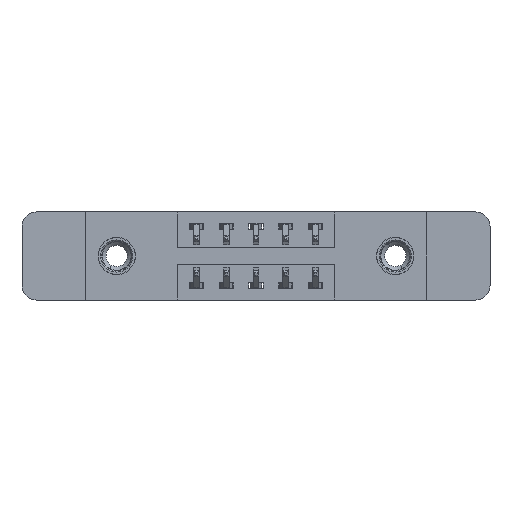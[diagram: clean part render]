
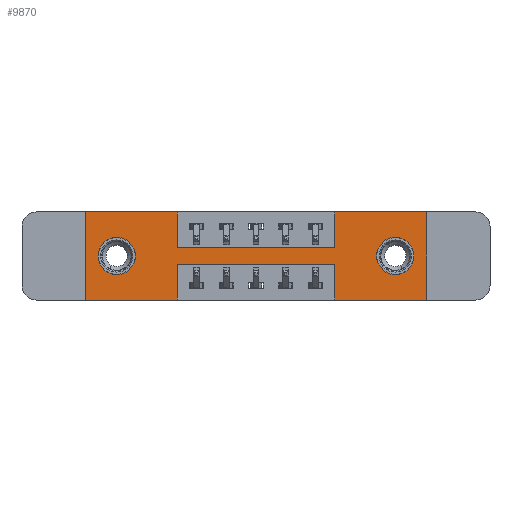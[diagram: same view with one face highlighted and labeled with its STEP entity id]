
A CAD part, front view. The second image highlights one B-rep face of the part: STEP entity #9870.
In plain terms, the highlighted planar face has unit normal (0, -1, 0).
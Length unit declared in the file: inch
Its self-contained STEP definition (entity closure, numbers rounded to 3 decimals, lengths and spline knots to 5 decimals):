
#35 = EDGE_LOOP ( 'NONE', ( #2740, #10334 ) ) ;
#72 = CARTESIAN_POINT ( 'NONE',  ( 0.3875, 0., -0.15 ) ) ;
#193 = CARTESIAN_POINT ( 'NONE',  ( 0.3875, 0., -0.22 ) ) ;
#396 = ORIENTED_EDGE ( 'NONE', *, *, #1984, .F. ) ;
#476 = DIRECTION ( 'NONE',  ( 0., 0., -1. ) ) ;
#534 = CIRCLE ( 'NONE', #6243, 0.078 ) ;
#608 = VERTEX_POINT ( 'NONE', #13250 ) ;
#846 = CARTESIAN_POINT ( 'NONE',  ( 0.1325, 0., -0.185 ) ) ;
#863 = DIRECTION ( 'NONE',  ( 0., 1., 0. ) ) ;
#986 = DIRECTION ( 'NONE',  ( 0., 0., 1. ) ) ;
#996 = CARTESIAN_POINT ( 'NONE',  ( 0.3875, 0., -0.22 ) ) ;
#1038 = DIRECTION ( 'NONE',  ( 0., 0., 1. ) ) ;
#1361 = CIRCLE ( 'NONE', #12333, 0.078 ) ;
#1553 = VERTEX_POINT ( 'NONE', #3649 ) ;
#1603 = DIRECTION ( 'NONE',  ( 0., 0., -1. ) ) ;
#1621 = CARTESIAN_POINT ( 'NONE',  ( 1.3025, 0., -0.107 ) ) ;
#1644 = CIRCLE ( 'NONE', #8771, 0.078 ) ;
#1811 = CARTESIAN_POINT ( 'NONE',  ( 1.3025, 0., -0.185 ) ) ;
#1864 = LINE ( 'NONE', #72, #11536 ) ;
#1931 = DIRECTION ( 'NONE',  ( 0., 0., 1. ) ) ;
#1952 = DIRECTION ( 'NONE',  ( 0., 0., -1. ) ) ;
#1984 = EDGE_CURVE ( 'NONE', #9420, #6050, #1864, .T. ) ;
#1992 = VECTOR ( 'NONE', #13668, 39.37008 ) ;
#2004 = ORIENTED_EDGE ( 'NONE', *, *, #5840, .F. ) ;
#2043 = DIRECTION ( 'NONE',  ( 0., -1., 0. ) ) ;
#2082 = VECTOR ( 'NONE', #986, 39.37008 ) ;
#2138 = VERTEX_POINT ( 'NONE', #6791 ) ;
#2183 = CARTESIAN_POINT ( 'NONE',  ( 1.435, 0., 0. ) ) ;
#2207 = ORIENTED_EDGE ( 'NONE', *, *, #3725, .F. ) ;
#2288 = DIRECTION ( 'NONE',  ( -1., 0., 0. ) ) ;
#2320 = CIRCLE ( 'NONE', #6111, 0.078 ) ;
#2337 = LINE ( 'NONE', #5996, #3648 ) ;
#2481 = EDGE_CURVE ( 'NONE', #6923, #7550, #2320, .T. ) ;
#2562 = CARTESIAN_POINT ( 'NONE',  ( 0.3875, 0., -0.37 ) ) ;
#2632 = VECTOR ( 'NONE', #2288, 39.37008 ) ;
#2740 = ORIENTED_EDGE ( 'NONE', *, *, #7923, .T. ) ;
#2781 = ORIENTED_EDGE ( 'NONE', *, *, #2481, .T. ) ;
#2967 = CARTESIAN_POINT ( 'NONE',  ( 0., 0., -0.37 ) ) ;
#2989 = DIRECTION ( 'NONE',  ( 0., 1., 0. ) ) ;
#3076 = CARTESIAN_POINT ( 'NONE',  ( 1.0475, 0., 0. ) ) ;
#3081 = VECTOR ( 'NONE', #7349, 39.37008 ) ;
#3181 = EDGE_CURVE ( 'NONE', #3489, #5596, #11012, .T. ) ;
#3206 = EDGE_CURVE ( 'NONE', #10962, #3489, #13653, .T. ) ;
#3361 = VERTEX_POINT ( 'NONE', #11330 ) ;
#3489 = VERTEX_POINT ( 'NONE', #10320 ) ;
#3536 = EDGE_CURVE ( 'NONE', #2138, #1553, #1644, .T. ) ;
#3585 = ORIENTED_EDGE ( 'NONE', *, *, #10074, .F. ) ;
#3632 = CARTESIAN_POINT ( 'NONE',  ( 1.0475, 0., -0.37 ) ) ;
#3648 = VECTOR ( 'NONE', #9548, 39.37008 ) ;
#3649 = CARTESIAN_POINT ( 'NONE',  ( 0.1325, 0., -0.107 ) ) ;
#3725 = EDGE_CURVE ( 'NONE', #5596, #3361, #4561, .T. ) ;
#3727 = CARTESIAN_POINT ( 'NONE',  ( 1.435, 0., -0.37 ) ) ;
#4040 = ORIENTED_EDGE ( 'NONE', *, *, #11218, .F. ) ;
#4129 = DIRECTION ( 'NONE',  ( 0., 0., -1. ) ) ;
#4209 = FACE_BOUND ( 'NONE', #35, .T. ) ;
#4561 = LINE ( 'NONE', #8550, #2632 ) ;
#4658 = CARTESIAN_POINT ( 'NONE',  ( 1.3025, 0., -0.185 ) ) ;
#4792 = ORIENTED_EDGE ( 'NONE', *, *, #5537, .F. ) ;
#4865 = VERTEX_POINT ( 'NONE', #9710 ) ;
#5009 = LINE ( 'NONE', #5022, #8159 ) ;
#5022 = CARTESIAN_POINT ( 'NONE',  ( 0., 0., -0.37 ) ) ;
#5079 = ORIENTED_EDGE ( 'NONE', *, *, #3181, .F. ) ;
#5196 = FACE_BOUND ( 'NONE', #7046, .T. ) ;
#5537 = EDGE_CURVE ( 'NONE', #3361, #13341, #12727, .T. ) ;
#5596 = VERTEX_POINT ( 'NONE', #3727 ) ;
#5840 = EDGE_CURVE ( 'NONE', #13059, #9420, #2337, .T. ) ;
#5899 = ORIENTED_EDGE ( 'NONE', *, *, #9355, .T. ) ;
#5996 = CARTESIAN_POINT ( 'NONE',  ( 0.3875, 0., 0. ) ) ;
#6050 = VERTEX_POINT ( 'NONE', #10403 ) ;
#6111 = AXIS2_PLACEMENT_3D ( 'NONE', #4658, #13098, #476 ) ;
#6243 = AXIS2_PLACEMENT_3D ( 'NONE', #1811, #863, #1952 ) ;
#6329 = DIRECTION ( 'NONE',  ( 1., 0., 0. ) ) ;
#6667 = FACE_OUTER_BOUND ( 'NONE', #9394, .T. ) ;
#6693 = VECTOR ( 'NONE', #6872, 39.37008 ) ;
#6791 = CARTESIAN_POINT ( 'NONE',  ( 0.1325, 0., -0.263 ) ) ;
#6872 = DIRECTION ( 'NONE',  ( 1., 0., 0. ) ) ;
#6923 = VERTEX_POINT ( 'NONE', #1621 ) ;
#6933 = DIRECTION ( 'NONE',  ( 0., 0., 1. ) ) ;
#7046 = EDGE_LOOP ( 'NONE', ( #2781, #5899 ) ) ;
#7098 = DIRECTION ( 'NONE',  ( -1., 0., 0. ) ) ;
#7129 = VECTOR ( 'NONE', #10797, 39.37008 ) ;
#7195 = EDGE_CURVE ( 'NONE', #9984, #7968, #10775, .T. ) ;
#7349 = DIRECTION ( 'NONE',  ( -1., 0., 0. ) ) ;
#7361 = DIRECTION ( 'NONE',  ( 0., 1., 0. ) ) ;
#7550 = VERTEX_POINT ( 'NONE', #12166 ) ;
#7695 = LINE ( 'NONE', #996, #3081 ) ;
#7807 = ORIENTED_EDGE ( 'NONE', *, *, #8978, .F. ) ;
#7821 = CARTESIAN_POINT ( 'NONE',  ( 0., 0., 0. ) ) ;
#7923 = EDGE_CURVE ( 'NONE', #1553, #2138, #1361, .T. ) ;
#7968 = VERTEX_POINT ( 'NONE', #10391 ) ;
#8159 = VECTOR ( 'NONE', #7098, 39.37008 ) ;
#8326 = AXIS2_PLACEMENT_3D ( 'NONE', #2967, #2043, #4129 ) ;
#8468 = CARTESIAN_POINT ( 'NONE',  ( 0.3875, 0., 0. ) ) ;
#8489 = LINE ( 'NONE', #3076, #2082 ) ;
#8550 = CARTESIAN_POINT ( 'NONE',  ( 0., 0., -0.37 ) ) ;
#8718 = VECTOR ( 'NONE', #6329, 39.37008 ) ;
#8771 = AXIS2_PLACEMENT_3D ( 'NONE', #13519, #7361, #1038 ) ;
#8876 = CARTESIAN_POINT ( 'NONE',  ( 1.0475, 0., 0. ) ) ;
#8887 = EDGE_CURVE ( 'NONE', #7968, #608, #5009, .T. ) ;
#8934 = CARTESIAN_POINT ( 'NONE',  ( 0., 0., 0. ) ) ;
#8978 = EDGE_CURVE ( 'NONE', #6050, #10962, #8489, .T. ) ;
#9051 = VECTOR ( 'NONE', #6933, 39.37008 ) ;
#9355 = EDGE_CURVE ( 'NONE', #7550, #6923, #534, .T. ) ;
#9394 = EDGE_LOOP ( 'NONE', ( #9949, #4040, #4792, #2207, #5079, #10603, #7807, #396, #2004, #13386, #3585, #10153 ) ) ;
#9420 = VERTEX_POINT ( 'NONE', #13679 ) ;
#9495 = LINE ( 'NONE', #8934, #6693 ) ;
#9548 = DIRECTION ( 'NONE',  ( 0., 0., -1. ) ) ;
#9678 = EDGE_CURVE ( 'NONE', #4865, #13059, #9495, .T. ) ;
#9710 = CARTESIAN_POINT ( 'NONE',  ( 0., 0., 0. ) ) ;
#9870 = ADVANCED_FACE ( 'NONE', ( #5196, #4209, #6667 ), #11474, .T. ) ;
#9949 = ORIENTED_EDGE ( 'NONE', *, *, #7195, .F. ) ;
#9984 = VERTEX_POINT ( 'NONE', #193 ) ;
#10074 = EDGE_CURVE ( 'NONE', #608, #4865, #11506, .T. ) ;
#10153 = ORIENTED_EDGE ( 'NONE', *, *, #8887, .F. ) ;
#10320 = CARTESIAN_POINT ( 'NONE',  ( 1.435, 0., 0. ) ) ;
#10334 = ORIENTED_EDGE ( 'NONE', *, *, #3536, .T. ) ;
#10391 = CARTESIAN_POINT ( 'NONE',  ( 0.3875, 0., -0.37 ) ) ;
#10403 = CARTESIAN_POINT ( 'NONE',  ( 1.0475, 0., -0.15 ) ) ;
#10603 = ORIENTED_EDGE ( 'NONE', *, *, #3206, .F. ) ;
#10775 = LINE ( 'NONE', #2562, #13617 ) ;
#10797 = DIRECTION ( 'NONE',  ( 0., 0., 1. ) ) ;
#10962 = VERTEX_POINT ( 'NONE', #8876 ) ;
#11012 = LINE ( 'NONE', #2183, #1992 ) ;
#11218 = EDGE_CURVE ( 'NONE', #13341, #9984, #7695, .T. ) ;
#11330 = CARTESIAN_POINT ( 'NONE',  ( 1.0475, 0., -0.37 ) ) ;
#11474 = PLANE ( 'NONE',  #8326 ) ;
#11506 = LINE ( 'NONE', #7821, #9051 ) ;
#11536 = VECTOR ( 'NONE', #12663, 39.37008 ) ;
#12166 = CARTESIAN_POINT ( 'NONE',  ( 1.3025, 0., -0.263 ) ) ;
#12333 = AXIS2_PLACEMENT_3D ( 'NONE', #846, #2989, #1931 ) ;
#12657 = CARTESIAN_POINT ( 'NONE',  ( 0., 0., 0. ) ) ;
#12663 = DIRECTION ( 'NONE',  ( 1., 0., 0. ) ) ;
#12727 = LINE ( 'NONE', #3632, #7129 ) ;
#12828 = CARTESIAN_POINT ( 'NONE',  ( 1.0475, 0., -0.22 ) ) ;
#13059 = VERTEX_POINT ( 'NONE', #8468 ) ;
#13098 = DIRECTION ( 'NONE',  ( 0., 1., 0. ) ) ;
#13250 = CARTESIAN_POINT ( 'NONE',  ( 0., 0., -0.37 ) ) ;
#13341 = VERTEX_POINT ( 'NONE', #12828 ) ;
#13386 = ORIENTED_EDGE ( 'NONE', *, *, #9678, .F. ) ;
#13519 = CARTESIAN_POINT ( 'NONE',  ( 0.1325, 0., -0.185 ) ) ;
#13617 = VECTOR ( 'NONE', #1603, 39.37008 ) ;
#13653 = LINE ( 'NONE', #12657, #8718 ) ;
#13668 = DIRECTION ( 'NONE',  ( 0., 0., -1. ) ) ;
#13679 = CARTESIAN_POINT ( 'NONE',  ( 0.3875, 0., -0.15 ) ) ;
